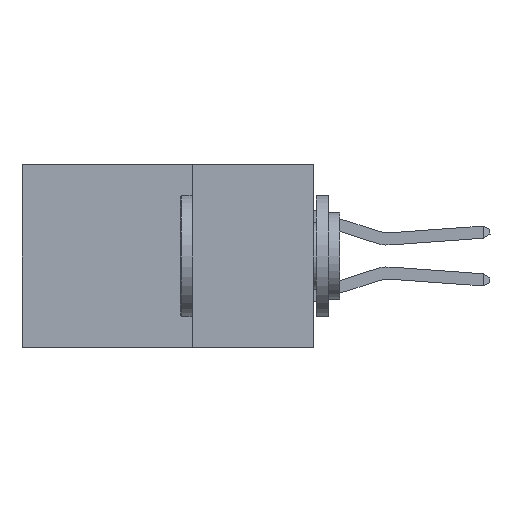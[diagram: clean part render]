
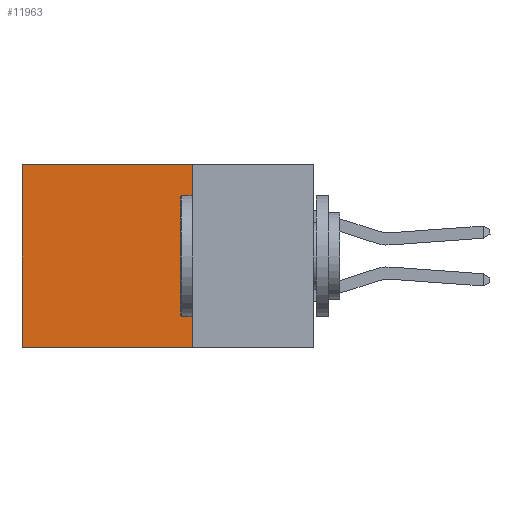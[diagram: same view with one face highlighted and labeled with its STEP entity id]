
A CAD part, left-side view. The second image highlights one B-rep face of the part: STEP entity #11963.
In plain terms, the highlighted planar face has unit normal (-1, 0, 0).
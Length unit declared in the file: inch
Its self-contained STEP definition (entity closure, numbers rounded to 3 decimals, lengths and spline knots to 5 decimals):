
#1018 = ORIENTED_EDGE ( 'NONE', *, *, #17413, .F. ) ;
#1190 = CARTESIAN_POINT ( 'NONE',  ( 0.2875, 0.25, -0.375 ) ) ;
#1462 = DIRECTION ( 'NONE',  ( 0., 1., 0. ) ) ;
#1575 = DIRECTION ( 'NONE',  ( 1., 0., 0. ) ) ;
#1888 = EDGE_CURVE ( 'NONE', #20173, #11174, #11168, .T. ) ;
#1980 = CARTESIAN_POINT ( 'NONE',  ( 0.2875, 0.25, 0. ) ) ;
#2748 = VECTOR ( 'NONE', #1462, 39.37008 ) ;
#5347 = CARTESIAN_POINT ( 'NONE',  ( 0.2875, 0.25, -0.375 ) ) ;
#5463 = LINE ( 'NONE', #6725, #2748 ) ;
#5596 = ORIENTED_EDGE ( 'NONE', *, *, #5705, .T. ) ;
#5705 = EDGE_CURVE ( 'NONE', #15889, #20173, #19980, .T. ) ;
#6588 = EDGE_LOOP ( 'NONE', ( #12111, #1018, #17167, #5596 ) ) ;
#6668 = VERTEX_POINT ( 'NONE', #5347 ) ;
#6725 = CARTESIAN_POINT ( 'NONE',  ( 0.2875, 0.25, -0.375 ) ) ;
#8738 = VECTOR ( 'NONE', #17964, 39.37008 ) ;
#9565 = DIRECTION ( 'NONE',  ( 0., 0., -1. ) ) ;
#10012 = VECTOR ( 'NONE', #17832, 39.37008 ) ;
#11007 = CARTESIAN_POINT ( 'NONE',  ( 0.2875, 0.6, -0.375 ) ) ;
#11168 = LINE ( 'NONE', #14448, #8738 ) ;
#11174 = VERTEX_POINT ( 'NONE', #11007 ) ;
#11921 = FACE_OUTER_BOUND ( 'NONE', #6588, .T. ) ;
#11963 = ADVANCED_FACE ( 'NONE', ( #11921 ), #14477, .F. ) ;
#12111 = ORIENTED_EDGE ( 'NONE', *, *, #1888, .T. ) ;
#12238 = CARTESIAN_POINT ( 'NONE',  ( 0.2875, 0.6, 0. ) ) ;
#14144 = DIRECTION ( 'NONE',  ( 0., 1., 0. ) ) ;
#14448 = CARTESIAN_POINT ( 'NONE',  ( 0.2875, 0.6, -0.375 ) ) ;
#14477 = PLANE ( 'NONE',  #21590 ) ;
#15889 = VERTEX_POINT ( 'NONE', #20684 ) ;
#17167 = ORIENTED_EDGE ( 'NONE', *, *, #19357, .F. ) ;
#17413 = EDGE_CURVE ( 'NONE', #6668, #11174, #5463, .T. ) ;
#17678 = CARTESIAN_POINT ( 'NONE',  ( 0.2875, 0.25, -0.375 ) ) ;
#17832 = DIRECTION ( 'NONE',  ( 0., 0., -1. ) ) ;
#17964 = DIRECTION ( 'NONE',  ( 0., 0., -1. ) ) ;
#18063 = VECTOR ( 'NONE', #14144, 39.37008 ) ;
#19357 = EDGE_CURVE ( 'NONE', #15889, #6668, #22283, .T. ) ;
#19980 = LINE ( 'NONE', #1980, #18063 ) ;
#20173 = VERTEX_POINT ( 'NONE', #12238 ) ;
#20684 = CARTESIAN_POINT ( 'NONE',  ( 0.2875, 0.25, 0. ) ) ;
#21590 = AXIS2_PLACEMENT_3D ( 'NONE', #1190, #1575, #9565 ) ;
#22283 = LINE ( 'NONE', #17678, #10012 ) ;
